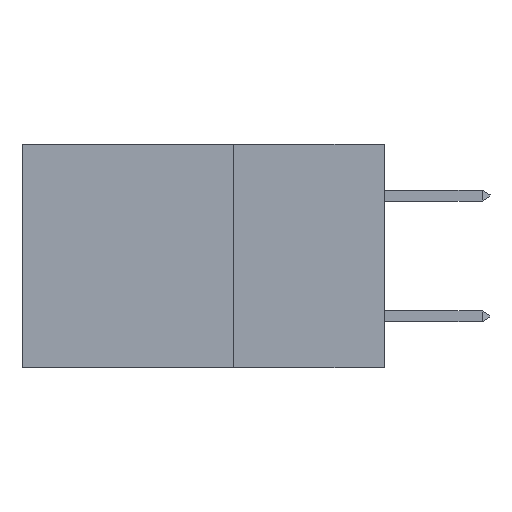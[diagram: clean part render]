
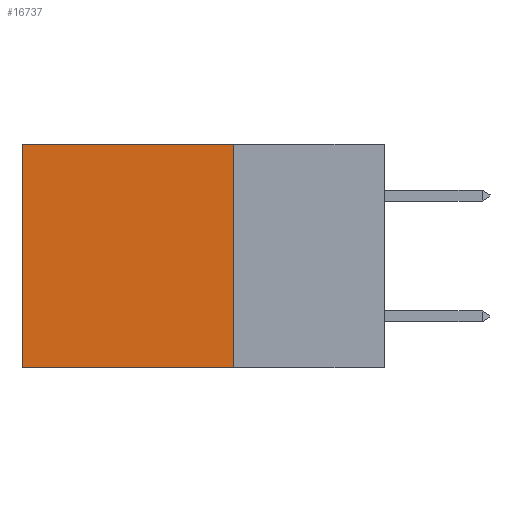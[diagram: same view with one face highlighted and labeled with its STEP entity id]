
A CAD part, left-side view. The second image highlights one B-rep face of the part: STEP entity #16737.
In plain terms, the highlighted planar face has unit normal (-1, 0, 0).
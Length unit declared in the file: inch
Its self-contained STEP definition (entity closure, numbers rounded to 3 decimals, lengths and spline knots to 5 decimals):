
#1036 = AXIS2_PLACEMENT_3D ( 'NONE', #15329, #6003, #18615 ) ;
#1149 = CARTESIAN_POINT ( 'NONE',  ( 0.2875, 0.6, 0. ) ) ;
#2366 = ORIENTED_EDGE ( 'NONE', *, *, #3120, .F. ) ;
#3120 = EDGE_CURVE ( 'NONE', #17156, #5773, #10000, .T. ) ;
#3974 = EDGE_CURVE ( 'NONE', #18777, #15998, #16429, .T. ) ;
#4128 = CARTESIAN_POINT ( 'NONE',  ( 0.2875, 0.25, 0. ) ) ;
#4232 = ORIENTED_EDGE ( 'NONE', *, *, #19006, .F. ) ;
#4697 = VECTOR ( 'NONE', #15169, 39.37008 ) ;
#4994 = CARTESIAN_POINT ( 'NONE',  ( 0.2875, 0.25, -0.37 ) ) ;
#5773 = VERTEX_POINT ( 'NONE', #9106 ) ;
#6003 = DIRECTION ( 'NONE',  ( 1., 0., 0. ) ) ;
#7079 = EDGE_LOOP ( 'NONE', ( #12005, #2366, #4232, #13059 ) ) ;
#7296 = VECTOR ( 'NONE', #11505, 39.37008 ) ;
#7692 = PLANE ( 'NONE',  #1036 ) ;
#8575 = CARTESIAN_POINT ( 'NONE',  ( 0.2875, 0.25, -0.37 ) ) ;
#8746 = CARTESIAN_POINT ( 'NONE',  ( 0.2875, 0.25, 0. ) ) ;
#9106 = CARTESIAN_POINT ( 'NONE',  ( 0.2875, 0.6, -0.37 ) ) ;
#9560 = EDGE_CURVE ( 'NONE', #15998, #5773, #14232, .T. ) ;
#10000 = LINE ( 'NONE', #4994, #7296 ) ;
#11329 = VECTOR ( 'NONE', #12234, 39.37008 ) ;
#11505 = DIRECTION ( 'NONE',  ( 0., 1., 0. ) ) ;
#11755 = LINE ( 'NONE', #15425, #4697 ) ;
#12005 = ORIENTED_EDGE ( 'NONE', *, *, #9560, .T. ) ;
#12234 = DIRECTION ( 'NONE',  ( 0., 0., -1. ) ) ;
#13059 = ORIENTED_EDGE ( 'NONE', *, *, #3974, .T. ) ;
#14232 = LINE ( 'NONE', #15302, #11329 ) ;
#14988 = DIRECTION ( 'NONE',  ( 0., 1., 0. ) ) ;
#15169 = DIRECTION ( 'NONE',  ( 0., 0., -1. ) ) ;
#15302 = CARTESIAN_POINT ( 'NONE',  ( 0.2875, 0.6, 0. ) ) ;
#15329 = CARTESIAN_POINT ( 'NONE',  ( 0.2875, 0.25, 0. ) ) ;
#15425 = CARTESIAN_POINT ( 'NONE',  ( 0.2875, 0.25, 0. ) ) ;
#15433 = VECTOR ( 'NONE', #14988, 39.37008 ) ;
#15998 = VERTEX_POINT ( 'NONE', #1149 ) ;
#16429 = LINE ( 'NONE', #4128, #15433 ) ;
#16737 = ADVANCED_FACE ( 'NONE', ( #17674 ), #7692, .F. ) ;
#17156 = VERTEX_POINT ( 'NONE', #8575 ) ;
#17674 = FACE_OUTER_BOUND ( 'NONE', #7079, .T. ) ;
#18615 = DIRECTION ( 'NONE',  ( 0., 0., -1. ) ) ;
#18777 = VERTEX_POINT ( 'NONE', #8746 ) ;
#19006 = EDGE_CURVE ( 'NONE', #18777, #17156, #11755, .T. ) ;
